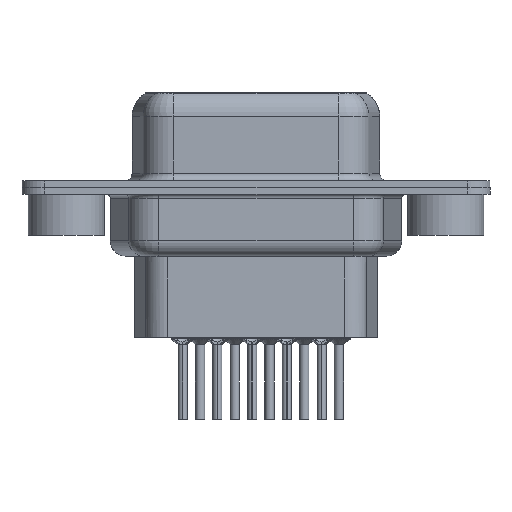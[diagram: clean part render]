
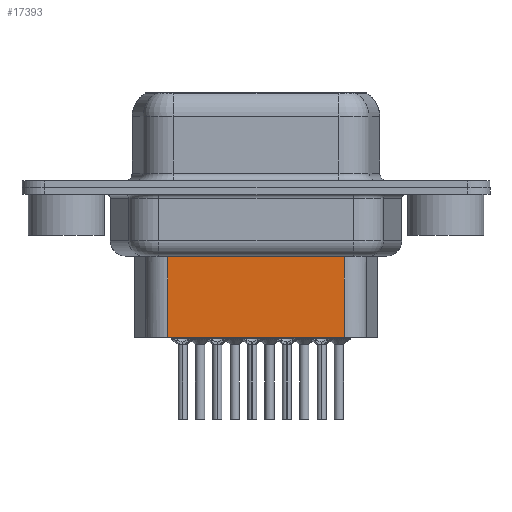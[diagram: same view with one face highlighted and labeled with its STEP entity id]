
A CAD part, front view. The second image highlights one B-rep face of the part: STEP entity #17393.
In plain terms, the highlighted planar face has unit normal (0, -1, 0).
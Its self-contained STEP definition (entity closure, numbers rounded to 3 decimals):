
#291 = DIRECTION ( 'NONE',  ( 1., 0., 0. ) ) ;
#1286 = CARTESIAN_POINT ( 'NONE',  ( 6.454, -3.5, -4.097 ) ) ;
#2373 = CARTESIAN_POINT ( 'NONE',  ( 6.701, -3.5, -3.1 ) ) ;
#2399 = VECTOR ( 'NONE', #8571, 1000. ) ;
#4105 = LINE ( 'NONE', #23373, #15033 ) ;
#4186 = LINE ( 'NONE', #1286, #20957 ) ;
#4399 = DIRECTION ( 'NONE',  ( 0., 0., -1. ) ) ;
#6734 = PLANE ( 'NONE',  #23869 ) ;
#7560 = ORIENTED_EDGE ( 'NONE', *, *, #28058, .T. ) ;
#7953 = EDGE_CURVE ( 'NONE', #15812, #17315, #19820, .T. ) ;
#8532 = CARTESIAN_POINT ( 'NONE',  ( 6.701, -3.5, -9.85 ) ) ;
#8554 = FACE_OUTER_BOUND ( 'NONE', #23273, .T. ) ;
#8571 = DIRECTION ( 'NONE',  ( -1., 0., 0. ) ) ;
#10249 = DIRECTION ( 'NONE',  ( 0., 0., -1. ) ) ;
#10318 = CARTESIAN_POINT ( 'NONE',  ( 18.289, -3.5, -9.85 ) ) ;
#11093 = CARTESIAN_POINT ( 'NONE',  ( 18.289, -3.5, -4.097 ) ) ;
#12104 = ORIENTED_EDGE ( 'NONE', *, *, #19844, .F. ) ;
#13316 = DIRECTION ( 'NONE',  ( 0., -1., 0. ) ) ;
#15033 = VECTOR ( 'NONE', #10249, 1000. ) ;
#15812 = VERTEX_POINT ( 'NONE', #10318 ) ;
#16313 = ORIENTED_EDGE ( 'NONE', *, *, #7953, .F. ) ;
#16509 = DIRECTION ( 'NONE',  ( -1., 0., 0. ) ) ;
#17315 = VERTEX_POINT ( 'NONE', #8532 ) ;
#17393 = ADVANCED_FACE ( 'NONE', ( #8554 ), #6734, .T. ) ;
#17487 = CARTESIAN_POINT ( 'NONE',  ( 18.289, -3.5, -3.1 ) ) ;
#17902 = CARTESIAN_POINT ( 'NONE',  ( 6.701, -3.5, -4.097 ) ) ;
#17968 = EDGE_CURVE ( 'NONE', #24780, #17315, #4105, .T. ) ;
#18447 = VECTOR ( 'NONE', #4399, 1000. ) ;
#19820 = LINE ( 'NONE', #23947, #2399 ) ;
#19844 = EDGE_CURVE ( 'NONE', #19903, #15812, #23607, .T. ) ;
#19903 = VERTEX_POINT ( 'NONE', #11093 ) ;
#20957 = VECTOR ( 'NONE', #16509, 1000. ) ;
#23273 = EDGE_LOOP ( 'NONE', ( #12104, #7560, #25801, #16313 ) ) ;
#23373 = CARTESIAN_POINT ( 'NONE',  ( 6.701, -3.5, -3.1 ) ) ;
#23607 = LINE ( 'NONE', #17487, #18447 ) ;
#23869 = AXIS2_PLACEMENT_3D ( 'NONE', #2373, #13316, #291 ) ;
#23947 = CARTESIAN_POINT ( 'NONE',  ( 6.701, -3.5, -9.85 ) ) ;
#24780 = VERTEX_POINT ( 'NONE', #17902 ) ;
#25801 = ORIENTED_EDGE ( 'NONE', *, *, #17968, .T. ) ;
#28058 = EDGE_CURVE ( 'NONE', #19903, #24780, #4186, .T. ) ;
